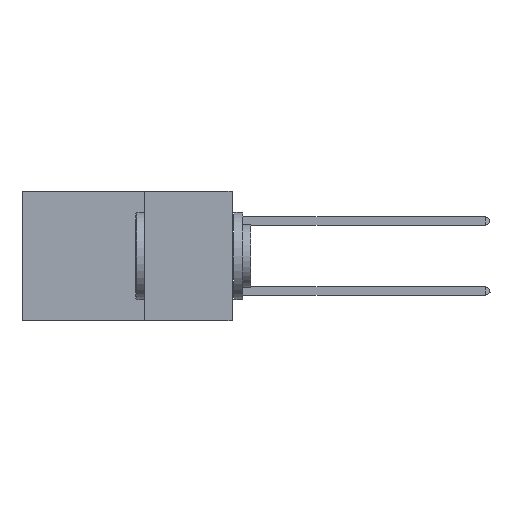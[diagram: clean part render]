
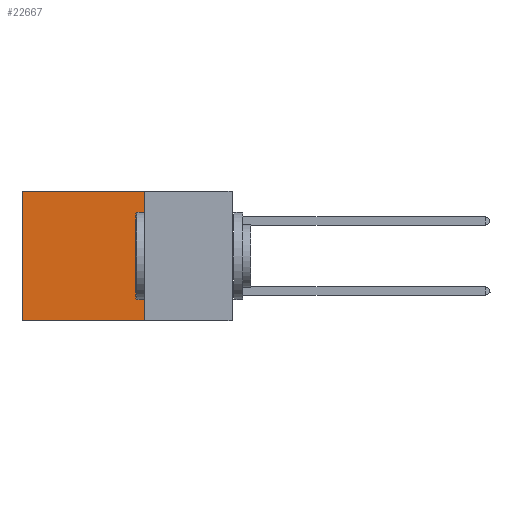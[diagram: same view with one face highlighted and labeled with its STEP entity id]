
A CAD part, left-side view. The second image highlights one B-rep face of the part: STEP entity #22667.
In plain terms, the highlighted planar face has unit normal (-1, 0, 0).
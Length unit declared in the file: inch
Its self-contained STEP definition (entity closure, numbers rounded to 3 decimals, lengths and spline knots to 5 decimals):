
#539 = LINE ( 'NONE', #8175, #8164 ) ;
#1072 = DIRECTION ( 'NONE',  ( 0., 0., -1. ) ) ;
#1209 = CARTESIAN_POINT ( 'NONE',  ( 0.2875, 0.6, -0.37 ) ) ;
#1237 = CARTESIAN_POINT ( 'NONE',  ( 0.2875, 0.6, 0. ) ) ;
#1642 = AXIS2_PLACEMENT_3D ( 'NONE', #5190, #19641, #10645 ) ;
#3064 = LINE ( 'NONE', #1237, #7305 ) ;
#3212 = LINE ( 'NONE', #13989, #16978 ) ;
#4356 = EDGE_CURVE ( 'NONE', #20286, #18637, #3212, .T. ) ;
#5047 = DIRECTION ( 'NONE',  ( 0., 0., -1. ) ) ;
#5190 = CARTESIAN_POINT ( 'NONE',  ( 0.2875, 0.25, 0. ) ) ;
#6793 = EDGE_CURVE ( 'NONE', #18637, #20865, #539, .T. ) ;
#7305 = VECTOR ( 'NONE', #1072, 39.37008 ) ;
#8164 = VECTOR ( 'NONE', #22434, 39.37008 ) ;
#8175 = CARTESIAN_POINT ( 'NONE',  ( 0.2875, 0.25, -0.37 ) ) ;
#8349 = CARTESIAN_POINT ( 'NONE',  ( 0.2875, 0.25, 0. ) ) ;
#8459 = EDGE_LOOP ( 'NONE', ( #9175, #15769, #18405, #18832 ) ) ;
#9175 = ORIENTED_EDGE ( 'NONE', *, *, #18872, .T. ) ;
#9300 = EDGE_CURVE ( 'NONE', #20286, #17311, #15072, .T. ) ;
#10645 = DIRECTION ( 'NONE',  ( 0., 0., -1. ) ) ;
#11022 = FACE_OUTER_BOUND ( 'NONE', #8459, .T. ) ;
#11376 = CARTESIAN_POINT ( 'NONE',  ( 0.2875, 0.25, 0. ) ) ;
#12580 = VECTOR ( 'NONE', #18627, 39.37008 ) ;
#13958 = CARTESIAN_POINT ( 'NONE',  ( 0.2875, 0.6, 0. ) ) ;
#13989 = CARTESIAN_POINT ( 'NONE',  ( 0.2875, 0.25, 0. ) ) ;
#14132 = PLANE ( 'NONE',  #1642 ) ;
#15072 = LINE ( 'NONE', #11376, #12580 ) ;
#15769 = ORIENTED_EDGE ( 'NONE', *, *, #6793, .F. ) ;
#16978 = VECTOR ( 'NONE', #5047, 39.37008 ) ;
#17311 = VERTEX_POINT ( 'NONE', #13958 ) ;
#18405 = ORIENTED_EDGE ( 'NONE', *, *, #4356, .F. ) ;
#18627 = DIRECTION ( 'NONE',  ( 0., 1., 0. ) ) ;
#18637 = VERTEX_POINT ( 'NONE', #18995 ) ;
#18832 = ORIENTED_EDGE ( 'NONE', *, *, #9300, .T. ) ;
#18872 = EDGE_CURVE ( 'NONE', #17311, #20865, #3064, .T. ) ;
#18995 = CARTESIAN_POINT ( 'NONE',  ( 0.2875, 0.25, -0.37 ) ) ;
#19641 = DIRECTION ( 'NONE',  ( 1., 0., 0. ) ) ;
#20286 = VERTEX_POINT ( 'NONE', #8349 ) ;
#20865 = VERTEX_POINT ( 'NONE', #1209 ) ;
#22434 = DIRECTION ( 'NONE',  ( 0., 1., 0. ) ) ;
#22667 = ADVANCED_FACE ( 'NONE', ( #11022 ), #14132, .F. ) ;
